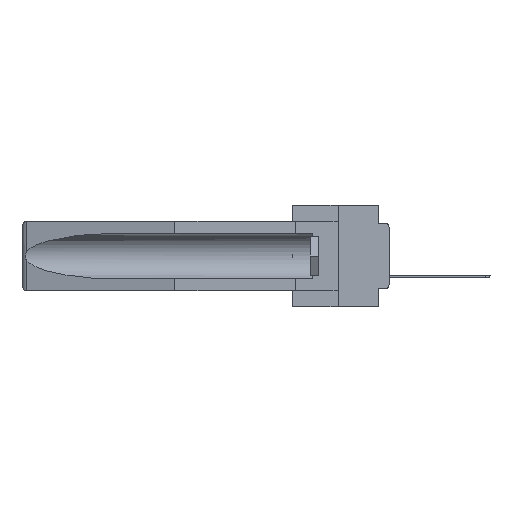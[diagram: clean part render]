
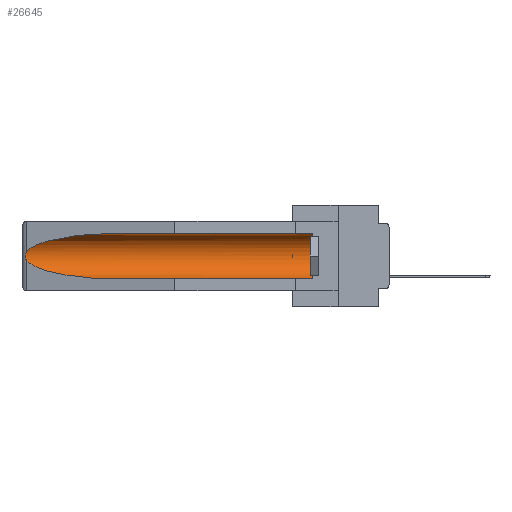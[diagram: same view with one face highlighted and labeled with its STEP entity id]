
A CAD part, left-side view. The second image highlights one B-rep face of the part: STEP entity #26645.
In plain terms, the highlighted cylindrical face has radius 2.857 mm (diameter 5.715 mm), a partial arc.
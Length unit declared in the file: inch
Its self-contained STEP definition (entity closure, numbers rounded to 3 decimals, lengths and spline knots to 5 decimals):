
#1076 = CYLINDRICAL_SURFACE ( 'NONE', #1892, 0.1125 ) ;
#1212 =( BOUNDED_CURVE ( )  B_SPLINE_CURVE ( 3, ( #39527, #11827, #24144, #11445 ),
 .UNSPECIFIED., .F., .F. ) 
 B_SPLINE_CURVE_WITH_KNOTS ( ( 4, 4 ),
 ( 4.71239, 6.08839 ),
 .UNSPECIFIED. ) 
 CURVE ( )  GEOMETRIC_REPRESENTATION_ITEM ( )  RATIONAL_B_SPLINE_CURVE ( ( 1., 0.848, 0.848, 1. ) ) 
 REPRESENTATION_ITEM ( '' )  );
#1892 = AXIS2_PLACEMENT_3D ( 'NONE', #4522, #37641, #28927 ) ;
#3107 = ORIENTED_EDGE ( 'NONE', *, *, #22757, .T. ) ;
#4275 = DIRECTION ( 'NONE',  ( 0., 1., 0. ) ) ;
#4522 = CARTESIAN_POINT ( 'NONE',  ( 0.155, -0.30754, -0.1715 ) ) ;
#4766 = CARTESIAN_POINT ( 'NONE',  ( 0.26597, 1.5296, -0.19026 ) ) ;
#5245 = CARTESIAN_POINT ( 'NONE',  ( 0.26537, 1.52718, -0.19328 ) ) ;
#7519 = DIRECTION ( 'NONE',  ( 0., 0., 1. ) ) ;
#7982 = CARTESIAN_POINT ( 'NONE',  ( 0.26597, 1.52961, -0.15275 ) ) ;
#8681 = CARTESIAN_POINT ( 'NONE',  ( 0.26537, 1.52718, -0.19328 ) ) ;
#8898 = ORIENTED_EDGE ( 'NONE', *, *, #18047, .T. ) ;
#9382 = VERTEX_POINT ( 'NONE', #39655 ) ;
#10695 = VERTEX_POINT ( 'NONE', #16242 ) ;
#11378 = CARTESIAN_POINT ( 'NONE',  ( 0.26654, 1.53092, -0.15636 ) ) ;
#11445 = CARTESIAN_POINT ( 'NONE',  ( 0.26537, 1.52718, -0.14972 ) ) ;
#11827 = CARTESIAN_POINT ( 'NONE',  ( 0.21114, 1.30732, -0.059 ) ) ;
#14210 = CARTESIAN_POINT ( 'NONE',  ( 0.2675, 1.53308, -0.17534 ) ) ;
#14932 = CARTESIAN_POINT ( 'NONE',  ( 0.25451, 1.48313, -0.24835 ) ) ;
#15485 = VECTOR ( 'NONE', #20325, 39.37008 ) ;
#16242 = CARTESIAN_POINT ( 'NONE',  ( 0.155, 1.07973, -0.284 ) ) ;
#16508 = CARTESIAN_POINT ( 'NONE',  ( 0.155, -0.30754, -0.284 ) ) ;
#16683 = VERTEX_POINT ( 'NONE', #22410 ) ;
#16782 = EDGE_CURVE ( 'NONE', #9382, #29217, #27029, .T. ) ;
#17427 = CARTESIAN_POINT ( 'NONE',  ( 0.26655, 1.53094, -0.18657 ) ) ;
#17679 =( BOUNDED_CURVE ( )  B_SPLINE_CURVE ( 3, ( #8681, #14932, #20965, #31091 ),
 .UNSPECIFIED., .F., .F. ) 
 B_SPLINE_CURVE_WITH_KNOTS ( ( 4, 4 ),
 ( 0.1948, 1.5708 ),
 .UNSPECIFIED. ) 
 CURVE ( )  GEOMETRIC_REPRESENTATION_ITEM ( )  RATIONAL_B_SPLINE_CURVE ( ( 1., 0.848, 0.848, 1. ) ) 
 REPRESENTATION_ITEM ( '' )  );
#18047 = EDGE_CURVE ( 'NONE', #16683, #30365, #1212, .T. ) ;
#20325 = DIRECTION ( 'NONE',  ( 0., 1., 0. ) ) ;
#20965 = CARTESIAN_POINT ( 'NONE',  ( 0.21114, 1.30732, -0.284 ) ) ;
#21988 = ORIENTED_EDGE ( 'NONE', *, *, #27040, .T. ) ;
#22329 = EDGE_LOOP ( 'NONE', ( #8898, #38901, #3107, #32054, #27429, #21988 ) ) ;
#22410 = CARTESIAN_POINT ( 'NONE',  ( 0.155, 1.07973, -0.059 ) ) ;
#22757 = EDGE_CURVE ( 'NONE', #30229, #10695, #17679, .T. ) ;
#24144 = CARTESIAN_POINT ( 'NONE',  ( 0.25451, 1.48313, -0.09465 ) ) ;
#25005 = EDGE_CURVE ( 'NONE', #30365, #30229, #32572, .T. ) ;
#25319 = CARTESIAN_POINT ( 'NONE',  ( 0.155, 0.126, -0.059 ) ) ;
#25498 = FACE_OUTER_BOUND ( 'NONE', #22329, .T. ) ;
#26205 = LINE ( 'NONE', #16508, #15485 ) ;
#26645 = ADVANCED_FACE ( 'NONE', ( #25498 ), #1076, .F. ) ;
#27029 = CIRCLE ( 'NONE', #34152, 0.1125 ) ;
#27040 = EDGE_CURVE ( 'NONE', #29217, #16683, #31507, .T. ) ;
#27429 = ORIENTED_EDGE ( 'NONE', *, *, #16782, .T. ) ;
#27683 = VECTOR ( 'NONE', #4275, 39.37008 ) ;
#27995 = CARTESIAN_POINT ( 'NONE',  ( 0.26537, 1.52718, -0.14972 ) ) ;
#28927 = DIRECTION ( 'NONE',  ( 0., 0., 1. ) ) ;
#29085 = CARTESIAN_POINT ( 'NONE',  ( 0.155, -0.30754, -0.059 ) ) ;
#29217 = VERTEX_POINT ( 'NONE', #25319 ) ;
#29947 = CARTESIAN_POINT ( 'NONE',  ( 0.2675, 1.53308, -0.16763 ) ) ;
#30140 = CARTESIAN_POINT ( 'NONE',  ( 0.26537, 1.52718, -0.14972 ) ) ;
#30229 = VERTEX_POINT ( 'NONE', #5245 ) ;
#30365 = VERTEX_POINT ( 'NONE', #27995 ) ;
#31091 = CARTESIAN_POINT ( 'NONE',  ( 0.155, 1.07973, -0.284 ) ) ;
#31507 = LINE ( 'NONE', #29085, #27683 ) ;
#32054 = ORIENTED_EDGE ( 'NONE', *, *, #35650, .F. ) ;
#32572 = B_SPLINE_CURVE_WITH_KNOTS ( 'NONE', 3,
 ( #30140, #7982, #11378, #36239, #29947, #14210, #33000, #17427, #4766, #38675 ),
 .UNSPECIFIED., .F., .F.,
 ( 4, 2, 2, 2, 4 ),
 ( 0., 0.00029, 0.00058, 0.00087, 0.00117 ),
 .UNSPECIFIED. ) ;
#33000 = CARTESIAN_POINT ( 'NONE',  ( 0.2673, 1.53269, -0.17917 ) ) ;
#34152 = AXIS2_PLACEMENT_3D ( 'NONE', #35575, #35370, #7519 ) ;
#35370 = DIRECTION ( 'NONE',  ( 0., -1., 0. ) ) ;
#35575 = CARTESIAN_POINT ( 'NONE',  ( 0.155, 0.126, -0.1715 ) ) ;
#35650 = EDGE_CURVE ( 'NONE', #9382, #10695, #26205, .T. ) ;
#36239 = CARTESIAN_POINT ( 'NONE',  ( 0.2673, 1.5327, -0.16383 ) ) ;
#37641 = DIRECTION ( 'NONE',  ( 0., 1., 0. ) ) ;
#38675 = CARTESIAN_POINT ( 'NONE',  ( 0.26537, 1.52718, -0.19328 ) ) ;
#38901 = ORIENTED_EDGE ( 'NONE', *, *, #25005, .T. ) ;
#39527 = CARTESIAN_POINT ( 'NONE',  ( 0.155, 1.07973, -0.059 ) ) ;
#39655 = CARTESIAN_POINT ( 'NONE',  ( 0.155, 0.126, -0.284 ) ) ;
